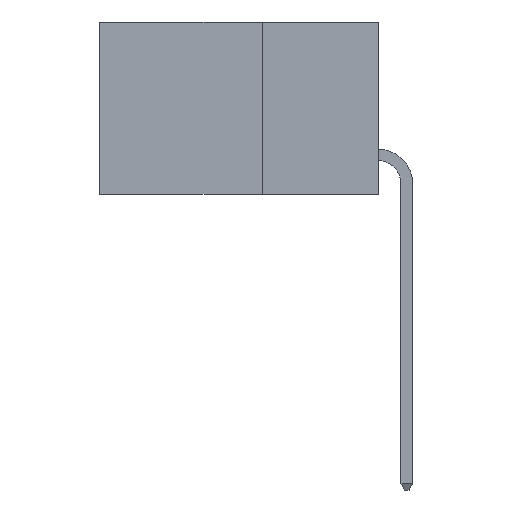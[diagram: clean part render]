
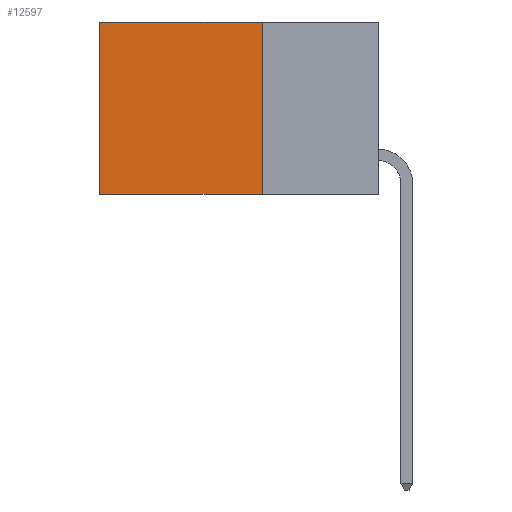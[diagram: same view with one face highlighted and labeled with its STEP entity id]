
A CAD part, left-side view. The second image highlights one B-rep face of the part: STEP entity #12597.
In plain terms, the highlighted planar face has unit normal (-1, 0, 0).
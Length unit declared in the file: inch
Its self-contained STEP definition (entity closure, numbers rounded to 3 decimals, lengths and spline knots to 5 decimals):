
#1035 = LINE ( 'NONE', #8198, #14200 ) ;
#2160 = FACE_OUTER_BOUND ( 'NONE', #11227, .T. ) ;
#2711 = VECTOR ( 'NONE', #10589, 39.37008 ) ;
#2731 = EDGE_CURVE ( 'NONE', #18991, #4505, #20665, .T. ) ;
#2778 = DIRECTION ( 'NONE',  ( 0., 1., 0. ) ) ;
#2876 = CARTESIAN_POINT ( 'NONE',  ( 0.2615, 0.25, -0.37 ) ) ;
#2944 = CARTESIAN_POINT ( 'NONE',  ( 0.2615, 0.25, 0. ) ) ;
#2954 = ORIENTED_EDGE ( 'NONE', *, *, #12882, .F. ) ;
#3443 = VECTOR ( 'NONE', #13077, 39.37008 ) ;
#4358 = VERTEX_POINT ( 'NONE', #7670 ) ;
#4376 = VECTOR ( 'NONE', #2778, 39.37008 ) ;
#4505 = VERTEX_POINT ( 'NONE', #4855 ) ;
#4713 = EDGE_CURVE ( 'NONE', #4505, #4358, #12571, .T. ) ;
#4855 = CARTESIAN_POINT ( 'NONE',  ( 0.2615, 0.6, 0. ) ) ;
#5698 = ORIENTED_EDGE ( 'NONE', *, *, #4713, .T. ) ;
#6829 = AXIS2_PLACEMENT_3D ( 'NONE', #10610, #10297, #10280 ) ;
#7582 = CARTESIAN_POINT ( 'NONE',  ( 0.2615, 0.25, 0. ) ) ;
#7670 = CARTESIAN_POINT ( 'NONE',  ( 0.2615, 0.6, -0.37 ) ) ;
#7734 = DIRECTION ( 'NONE',  ( 0., 0., -1. ) ) ;
#8198 = CARTESIAN_POINT ( 'NONE',  ( 0.2615, 0.25, -0.37 ) ) ;
#10280 = DIRECTION ( 'NONE',  ( 0., 0., -1. ) ) ;
#10297 = DIRECTION ( 'NONE',  ( 1., 0., 0. ) ) ;
#10425 = PLANE ( 'NONE',  #6829 ) ;
#10571 = ORIENTED_EDGE ( 'NONE', *, *, #2731, .T. ) ;
#10589 = DIRECTION ( 'NONE',  ( 0., 1., 0. ) ) ;
#10610 = CARTESIAN_POINT ( 'NONE',  ( 0.2615, 0.25, -0.37 ) ) ;
#11227 = EDGE_LOOP ( 'NONE', ( #5698, #11399, #2954, #10571 ) ) ;
#11399 = ORIENTED_EDGE ( 'NONE', *, *, #19018, .F. ) ;
#12571 = LINE ( 'NONE', #12954, #3443 ) ;
#12597 = ADVANCED_FACE ( 'NONE', ( #2160 ), #10425, .F. ) ;
#12882 = EDGE_CURVE ( 'NONE', #18991, #15205, #1035, .T. ) ;
#12954 = CARTESIAN_POINT ( 'NONE',  ( 0.2615, 0.6, -0.37 ) ) ;
#13077 = DIRECTION ( 'NONE',  ( 0., 0., -1. ) ) ;
#13311 = CARTESIAN_POINT ( 'NONE',  ( 0.2615, 0.25, -0.37 ) ) ;
#14200 = VECTOR ( 'NONE', #7734, 39.37008 ) ;
#15205 = VERTEX_POINT ( 'NONE', #13311 ) ;
#18991 = VERTEX_POINT ( 'NONE', #2944 ) ;
#19018 = EDGE_CURVE ( 'NONE', #15205, #4358, #21599, .T. ) ;
#20665 = LINE ( 'NONE', #7582, #2711 ) ;
#21599 = LINE ( 'NONE', #2876, #4376 ) ;
